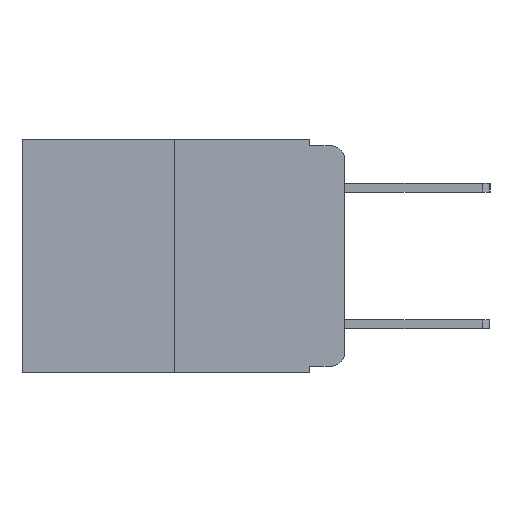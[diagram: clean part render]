
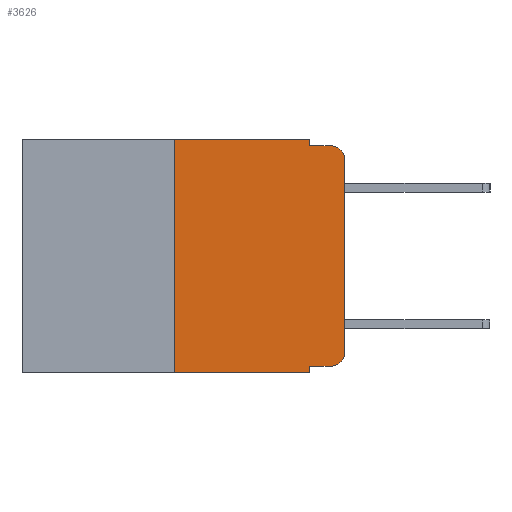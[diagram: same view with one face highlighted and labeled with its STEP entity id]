
A CAD part, left-side view. The second image highlights one B-rep face of the part: STEP entity #3626.
In plain terms, the highlighted planar face has unit normal (-1, 0, 0).
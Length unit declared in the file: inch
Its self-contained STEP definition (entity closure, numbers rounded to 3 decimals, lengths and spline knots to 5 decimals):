
#180 = DIRECTION ( 'NONE',  ( 0., 0., -1. ) ) ;
#412 = VERTEX_POINT ( 'NONE', #1008 ) ;
#478 = ORIENTED_EDGE ( 'NONE', *, *, #9495, .F. ) ;
#490 = ORIENTED_EDGE ( 'NONE', *, *, #11115, .T. ) ;
#828 = DIRECTION ( 'NONE',  ( 0., 0., 1. ) ) ;
#886 = VERTEX_POINT ( 'NONE', #8034 ) ;
#1008 = CARTESIAN_POINT ( 'NONE',  ( 0., 0., -0.03 ) ) ;
#1244 = DIRECTION ( 'NONE',  ( -1., 0., 0. ) ) ;
#1401 = DIRECTION ( 'NONE',  ( 0., 0., 1. ) ) ;
#1576 = VECTOR ( 'NONE', #1401, 39.37008 ) ;
#1589 = VECTOR ( 'NONE', #8825, 39.37008 ) ;
#1807 = VERTEX_POINT ( 'NONE', #8330 ) ;
#2260 = VECTOR ( 'NONE', #6644, 39.37008 ) ;
#2323 = CIRCLE ( 'NONE', #9126, 0.02 ) ;
#2447 = FACE_OUTER_BOUND ( 'NONE', #4406, .T. ) ;
#2905 = CARTESIAN_POINT ( 'NONE',  ( 0., 0.051, -0.333 ) ) ;
#3523 = DIRECTION ( 'NONE',  ( 0., -1., 0. ) ) ;
#3626 = ADVANCED_FACE ( 'NONE', ( #2447 ), #5410, .F. ) ;
#3826 = CARTESIAN_POINT ( 'NONE',  ( 0., 0.051, -0.333 ) ) ;
#3855 = CARTESIAN_POINT ( 'NONE',  ( 0., 0.051, -0.343 ) ) ;
#4130 = VERTEX_POINT ( 'NONE', #3855 ) ;
#4341 = CARTESIAN_POINT ( 'NONE',  ( 0., 0.051, 0. ) ) ;
#4406 = EDGE_LOOP ( 'NONE', ( #490, #7900, #10366, #478, #6165, #6454, #8688, #8945, #11346, #4883 ) ) ;
#4444 = VECTOR ( 'NONE', #5242, 39.37008 ) ;
#4821 = VECTOR ( 'NONE', #3523, 39.37008 ) ;
#4883 = ORIENTED_EDGE ( 'NONE', *, *, #7263, .T. ) ;
#5242 = DIRECTION ( 'NONE',  ( 0., 0., -1. ) ) ;
#5299 = CARTESIAN_POINT ( 'NONE',  ( 0., 0., -0.313 ) ) ;
#5410 = PLANE ( 'NONE',  #10385 ) ;
#5619 = CARTESIAN_POINT ( 'NONE',  ( 0., 0.051, -0.01 ) ) ;
#6165 = ORIENTED_EDGE ( 'NONE', *, *, #8869, .F. ) ;
#6171 = VERTEX_POINT ( 'NONE', #8269 ) ;
#6328 = DIRECTION ( 'NONE',  ( 1., 0., 0. ) ) ;
#6454 = ORIENTED_EDGE ( 'NONE', *, *, #8932, .F. ) ;
#6533 = CARTESIAN_POINT ( 'NONE',  ( 0., 0.25, 0. ) ) ;
#6582 = DIRECTION ( 'NONE',  ( -1., 0., 0. ) ) ;
#6607 = CARTESIAN_POINT ( 'NONE',  ( 0., 0.473, -0.343 ) ) ;
#6644 = DIRECTION ( 'NONE',  ( 0., -1., 0. ) ) ;
#6668 = DIRECTION ( 'NONE',  ( 0., -1., 0. ) ) ;
#7055 = VECTOR ( 'NONE', #828, 39.37008 ) ;
#7102 = LINE ( 'NONE', #2905, #11194 ) ;
#7197 = VECTOR ( 'NONE', #6668, 39.37008 ) ;
#7205 = LINE ( 'NONE', #10338, #4444 ) ;
#7213 = LINE ( 'NONE', #10624, #4821 ) ;
#7263 = EDGE_CURVE ( 'NONE', #886, #11295, #2323, .T. ) ;
#7266 = CARTESIAN_POINT ( 'NONE',  ( 0., 0.02, -0.313 ) ) ;
#7514 = CARTESIAN_POINT ( 'NONE',  ( 0., 0.051, -0.01 ) ) ;
#7817 = CARTESIAN_POINT ( 'NONE',  ( 0., 0.02, -0.01 ) ) ;
#7819 = EDGE_CURVE ( 'NONE', #9105, #886, #7102, .T. ) ;
#7900 = ORIENTED_EDGE ( 'NONE', *, *, #10586, .T. ) ;
#8034 = CARTESIAN_POINT ( 'NONE',  ( 0., 0.02, -0.333 ) ) ;
#8102 = DIRECTION ( 'NONE',  ( 0., 0., -1. ) ) ;
#8269 = CARTESIAN_POINT ( 'NONE',  ( 0., 0.051, 0. ) ) ;
#8330 = CARTESIAN_POINT ( 'NONE',  ( 0., 0.25, -0.343 ) ) ;
#8383 = EDGE_CURVE ( 'NONE', #9105, #4130, #11314, .T. ) ;
#8466 = DIRECTION ( 'NONE',  ( 0., -1., 0. ) ) ;
#8688 = ORIENTED_EDGE ( 'NONE', *, *, #11954, .T. ) ;
#8825 = DIRECTION ( 'NONE',  ( 0., 0., -1. ) ) ;
#8869 = EDGE_CURVE ( 'NONE', #10636, #6171, #7213, .T. ) ;
#8932 = EDGE_CURVE ( 'NONE', #1807, #10636, #11073, .T. ) ;
#8945 = ORIENTED_EDGE ( 'NONE', *, *, #8383, .F. ) ;
#9005 = LINE ( 'NONE', #11085, #7055 ) ;
#9105 = VERTEX_POINT ( 'NONE', #3826 ) ;
#9126 = AXIS2_PLACEMENT_3D ( 'NONE', #7266, #1244, #8102 ) ;
#9495 = EDGE_CURVE ( 'NONE', #6171, #11777, #7205, .T. ) ;
#9650 = LINE ( 'NONE', #6607, #2260 ) ;
#9893 = CIRCLE ( 'NONE', #10156, 0.02 ) ;
#10036 = EDGE_CURVE ( 'NONE', #11777, #11163, #11779, .T. ) ;
#10156 = AXIS2_PLACEMENT_3D ( 'NONE', #11484, #6582, #180 ) ;
#10338 = CARTESIAN_POINT ( 'NONE',  ( 0., 0.051, 0. ) ) ;
#10366 = ORIENTED_EDGE ( 'NONE', *, *, #10036, .F. ) ;
#10385 = AXIS2_PLACEMENT_3D ( 'NONE', #11274, #6328, #12050 ) ;
#10586 = EDGE_CURVE ( 'NONE', #412, #11163, #9893, .T. ) ;
#10624 = CARTESIAN_POINT ( 'NONE',  ( 0., 0.473, 0. ) ) ;
#10636 = VERTEX_POINT ( 'NONE', #11524 ) ;
#11073 = LINE ( 'NONE', #6533, #1576 ) ;
#11085 = CARTESIAN_POINT ( 'NONE',  ( 0., 0., 0. ) ) ;
#11115 = EDGE_CURVE ( 'NONE', #11295, #412, #9005, .T. ) ;
#11163 = VERTEX_POINT ( 'NONE', #7817 ) ;
#11194 = VECTOR ( 'NONE', #8466, 39.37008 ) ;
#11274 = CARTESIAN_POINT ( 'NONE',  ( 0., 0.473, 0. ) ) ;
#11295 = VERTEX_POINT ( 'NONE', #5299 ) ;
#11314 = LINE ( 'NONE', #4341, #1589 ) ;
#11346 = ORIENTED_EDGE ( 'NONE', *, *, #7819, .T. ) ;
#11484 = CARTESIAN_POINT ( 'NONE',  ( 0., 0.02, -0.03 ) ) ;
#11524 = CARTESIAN_POINT ( 'NONE',  ( 0., 0.25, 0. ) ) ;
#11777 = VERTEX_POINT ( 'NONE', #5619 ) ;
#11779 = LINE ( 'NONE', #7514, #7197 ) ;
#11954 = EDGE_CURVE ( 'NONE', #1807, #4130, #9650, .T. ) ;
#12050 = DIRECTION ( 'NONE',  ( 0., 0., -1. ) ) ;
